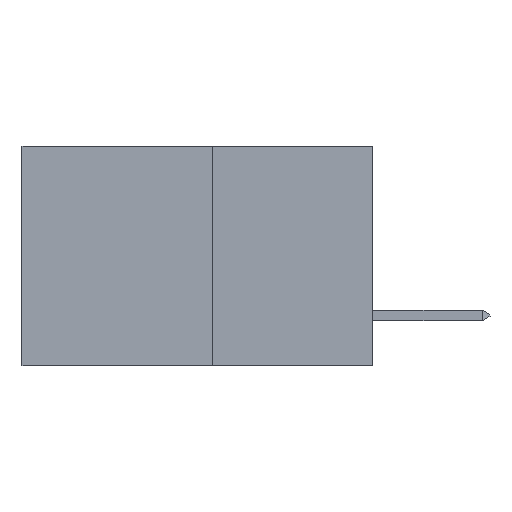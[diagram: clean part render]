
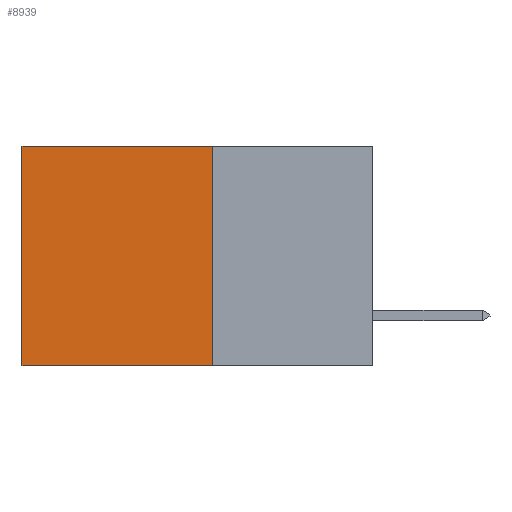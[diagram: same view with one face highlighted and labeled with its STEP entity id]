
A CAD part, left-side view. The second image highlights one B-rep face of the part: STEP entity #8939.
In plain terms, the highlighted planar face has unit normal (-1, 0, 0).
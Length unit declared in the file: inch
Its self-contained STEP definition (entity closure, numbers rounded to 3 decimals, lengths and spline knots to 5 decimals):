
#177 = EDGE_CURVE ( 'NONE', #5487, #10513, #10955, .T. ) ;
#590 = CARTESIAN_POINT ( 'NONE',  ( 0.277, 0.27, -0.37 ) ) ;
#972 = CARTESIAN_POINT ( 'NONE',  ( 0.277, 0.59, -0.37 ) ) ;
#1869 = CARTESIAN_POINT ( 'NONE',  ( 0.277, 0.27, -0.37 ) ) ;
#2054 = LINE ( 'NONE', #5955, #4613 ) ;
#2789 = DIRECTION ( 'NONE',  ( 0., 0., -1. ) ) ;
#3407 = EDGE_LOOP ( 'NONE', ( #9021, #11203, #4698, #6990 ) ) ;
#3913 = VERTEX_POINT ( 'NONE', #590 ) ;
#3945 = CARTESIAN_POINT ( 'NONE',  ( 0.277, 0.59, -0.37 ) ) ;
#4548 = FACE_OUTER_BOUND ( 'NONE', #3407, .T. ) ;
#4613 = VECTOR ( 'NONE', #6518, 39.37008 ) ;
#4698 = ORIENTED_EDGE ( 'NONE', *, *, #5400, .F. ) ;
#4729 = PLANE ( 'NONE',  #10181 ) ;
#4772 = EDGE_CURVE ( 'NONE', #3913, #10513, #9622, .T. ) ;
#4972 = VECTOR ( 'NONE', #9644, 39.37008 ) ;
#5400 = EDGE_CURVE ( 'NONE', #6648, #3913, #2054, .T. ) ;
#5487 = VERTEX_POINT ( 'NONE', #6056 ) ;
#5890 = CARTESIAN_POINT ( 'NONE',  ( 0.277, 0.27, 0. ) ) ;
#5955 = CARTESIAN_POINT ( 'NONE',  ( 0.277, 0.27, -0.37 ) ) ;
#6056 = CARTESIAN_POINT ( 'NONE',  ( 0.277, 0.59, 0. ) ) ;
#6192 = CARTESIAN_POINT ( 'NONE',  ( 0.277, 0.27, -0.37 ) ) ;
#6264 = DIRECTION ( 'NONE',  ( 0., 1., 0. ) ) ;
#6518 = DIRECTION ( 'NONE',  ( 0., 0., -1. ) ) ;
#6648 = VERTEX_POINT ( 'NONE', #5890 ) ;
#6990 = ORIENTED_EDGE ( 'NONE', *, *, #10948, .T. ) ;
#7073 = VECTOR ( 'NONE', #6264, 39.37008 ) ;
#7471 = DIRECTION ( 'NONE',  ( 0., 0., -1. ) ) ;
#8202 = DIRECTION ( 'NONE',  ( 1., 0., 0. ) ) ;
#8798 = CARTESIAN_POINT ( 'NONE',  ( 0.277, 0.27, 0. ) ) ;
#8939 = ADVANCED_FACE ( 'NONE', ( #4548 ), #4729, .F. ) ;
#9021 = ORIENTED_EDGE ( 'NONE', *, *, #177, .T. ) ;
#9622 = LINE ( 'NONE', #6192, #7073 ) ;
#9644 = DIRECTION ( 'NONE',  ( 0., 1., 0. ) ) ;
#10181 = AXIS2_PLACEMENT_3D ( 'NONE', #1869, #8202, #2789 ) ;
#10428 = VECTOR ( 'NONE', #7471, 39.37008 ) ;
#10513 = VERTEX_POINT ( 'NONE', #3945 ) ;
#10948 = EDGE_CURVE ( 'NONE', #6648, #5487, #11423, .T. ) ;
#10955 = LINE ( 'NONE', #972, #10428 ) ;
#11203 = ORIENTED_EDGE ( 'NONE', *, *, #4772, .F. ) ;
#11423 = LINE ( 'NONE', #8798, #4972 ) ;
